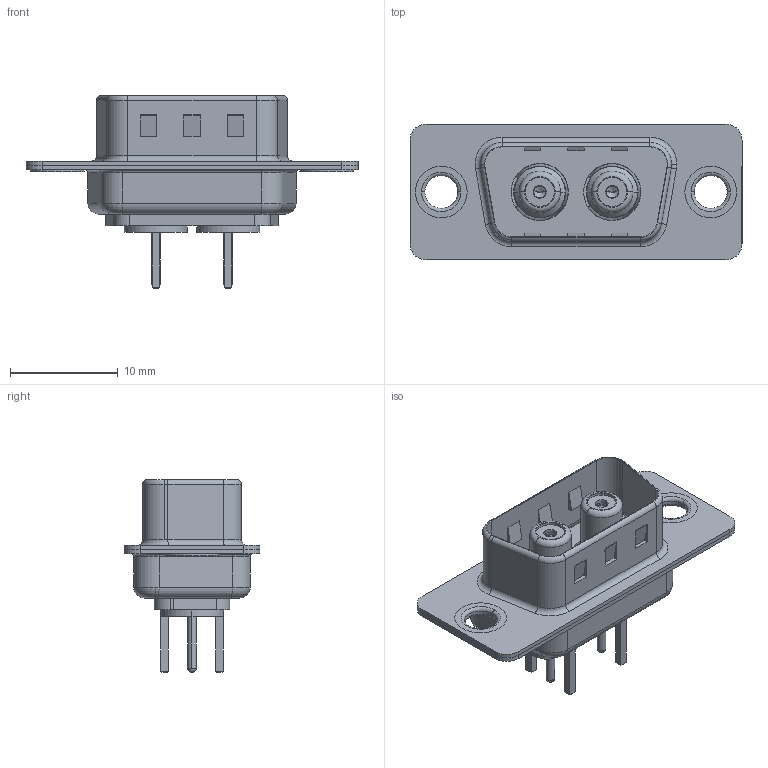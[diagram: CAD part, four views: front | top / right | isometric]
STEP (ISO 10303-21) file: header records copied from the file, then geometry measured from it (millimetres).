
FILE_DESCRIPTION (( 'STEP AP203' ), '1' );
FILE_NAME ('627-2W2-224-5T1.STEP', '2019-05-23T20:20:57', ( '' ), ( '' ), 'SwSTEP 2.0', 'SolidWorks 2016', '' );
FILE_SCHEMA (( 'CONFIG_CONTROL_DESIGN' ));
Length unit declared in the file: millimetre
Products named in the file (11): 627Combo Thru Hole Rivet; Co-Ax Jack_Straight PC Tail; Insulator Socket; Insulator Socket 2; Locking Collar; Socket_Str; 627Combo Housing_2W2; Co-Ax Jack Assy_S; 627Combo Shell Rear_09 Contacts; 627-2W2-224-5T1; 627Combo Shell Front_09 Contacts
Assembly tree (12 placements, depth 3):
  627-2W2-224-5T1
    627Combo Housing_2W2
    627Combo Shell Rear_09 Contacts
    627Combo Shell Front_09 Contacts
    627Combo Thru Hole Rivet  x2
    Co-Ax Jack Assy_S  x2
      Co-Ax Jack_Straight PC Tail
      Insulator Socket
      Insulator Socket 2
      Locking Collar
      Socket_Str
Bounding box: 30.8 x 12.6 x 17.9 mm (x, y, z)
Volume: 1279.5 mm3; surface area: 4255.4 mm2
Topology: 15 solids, 15 shells, 500 faces, 1173 edges, 730 vertices
Faces by surface type: cylinder 207, plane 201, torus 66, cone 18, bspline 4, sphere 4
Entity records: 12233 total; most frequent: DIRECTION 2044, CARTESIAN_POINT 1985, ORIENTED_EDGE 1780, EDGE_CURVE 890, AXIS2_PLACEMENT_3D 793, VERTEX_POINT 558, VECTOR 458, LINE 458
